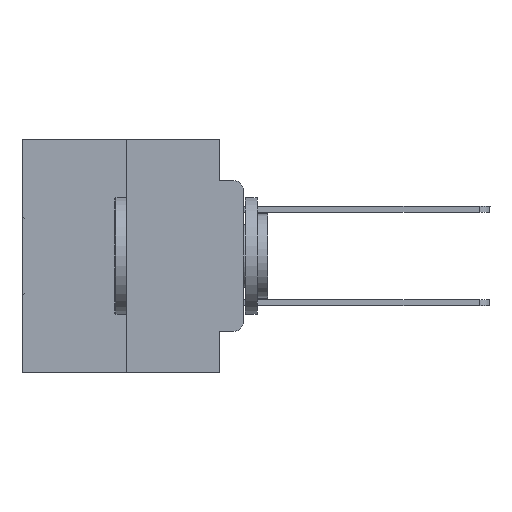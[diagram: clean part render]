
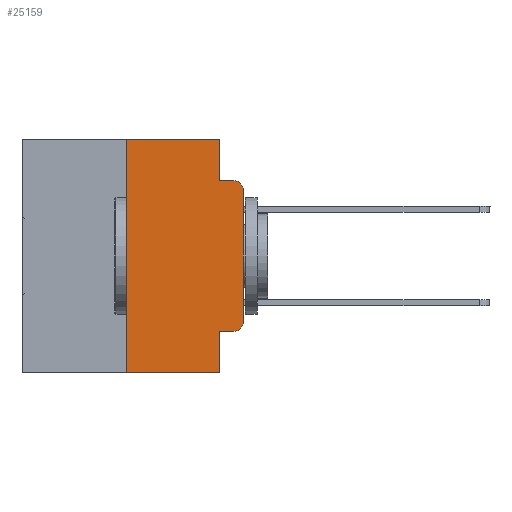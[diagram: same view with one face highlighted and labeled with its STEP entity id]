
A CAD part, left-side view. The second image highlights one B-rep face of the part: STEP entity #25159.
In plain terms, the highlighted planar face has unit normal (-1, 0, 0).
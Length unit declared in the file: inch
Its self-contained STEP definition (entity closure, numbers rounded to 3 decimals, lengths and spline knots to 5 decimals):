
#123 = ORIENTED_EDGE ( 'NONE', *, *, #10604, .T. ) ;
#193 = ORIENTED_EDGE ( 'NONE', *, *, #23013, .F. ) ;
#259 = ORIENTED_EDGE ( 'NONE', *, *, #24618, .F. ) ;
#698 = CARTESIAN_POINT ( 'NONE',  ( 0., 0., -0.3915 ) ) ;
#1073 = ORIENTED_EDGE ( 'NONE', *, *, #23435, .F. ) ;
#1440 = ORIENTED_EDGE ( 'NONE', *, *, #4378, .F. ) ;
#1446 = VERTEX_POINT ( 'NONE', #698 ) ;
#1528 = ORIENTED_EDGE ( 'NONE', *, *, #29023, .T. ) ;
#1640 = AXIS2_PLACEMENT_3D ( 'NONE', #9960, #26899, #12381 ) ;
#1668 = CARTESIAN_POINT ( 'NONE',  ( 0., 0.051, -0.4115 ) ) ;
#1795 = ORIENTED_EDGE ( 'NONE', *, *, #25644, .F. ) ;
#2915 = VERTEX_POINT ( 'NONE', #30179 ) ;
#3330 = CARTESIAN_POINT ( 'NONE',  ( 0., 0.473, 0. ) ) ;
#3555 = ORIENTED_EDGE ( 'NONE', *, *, #5461, .T. ) ;
#3593 = VERTEX_POINT ( 'NONE', #16585 ) ;
#3772 = ORIENTED_EDGE ( 'NONE', *, *, #14699, .T. ) ;
#4323 = DIRECTION ( 'NONE',  ( 0., -1., 0. ) ) ;
#4378 = EDGE_CURVE ( 'NONE', #27528, #13799, #26912, .T. ) ;
#4820 = CARTESIAN_POINT ( 'NONE',  ( 0., 0.051, -0.4115 ) ) ;
#5461 = EDGE_CURVE ( 'NONE', #28238, #3593, #11189, .T. ) ;
#5776 = DIRECTION ( 'NONE',  ( 0., -1., 0. ) ) ;
#5887 = DIRECTION ( 'NONE',  ( 0., 0., -1. ) ) ;
#6039 = DIRECTION ( 'NONE',  ( 0., 0., -1. ) ) ;
#6043 = VECTOR ( 'NONE', #5776, 39.37008 ) ;
#6338 = VECTOR ( 'NONE', #8781, 39.37008 ) ;
#6846 = DIRECTION ( 'NONE',  ( 0., -1., 0. ) ) ;
#6979 = CIRCLE ( 'NONE', #1640, 0.02 ) ;
#8599 = CARTESIAN_POINT ( 'NONE',  ( 0., 0.25, 0. ) ) ;
#8781 = DIRECTION ( 'NONE',  ( 0., 0., -1. ) ) ;
#8813 = DIRECTION ( 'NONE',  ( 0., 0., 1. ) ) ;
#9784 = FACE_OUTER_BOUND ( 'NONE', #12762, .T. ) ;
#9960 = CARTESIAN_POINT ( 'NONE',  ( 0., 0.02, -0.3915 ) ) ;
#10604 = EDGE_CURVE ( 'NONE', #21894, #22448, #30236, .T. ) ;
#10628 = CARTESIAN_POINT ( 'NONE',  ( 0., 0.473, -0.5 ) ) ;
#10688 = CARTESIAN_POINT ( 'NONE',  ( 0., 0., -0.1085 ) ) ;
#10834 = DIRECTION ( 'NONE',  ( 0., 0., 1. ) ) ;
#11189 = LINE ( 'NONE', #1668, #16890 ) ;
#11787 = LINE ( 'NONE', #22932, #23922 ) ;
#12381 = DIRECTION ( 'NONE',  ( 0., 0., -1. ) ) ;
#12550 = LINE ( 'NONE', #10628, #6043 ) ;
#12762 = EDGE_LOOP ( 'NONE', ( #30031, #123, #193, #259, #1073, #1440, #1528, #1795, #3555, #3772 ) ) ;
#13799 = VERTEX_POINT ( 'NONE', #21155 ) ;
#13917 = VECTOR ( 'NONE', #6039, 39.37008 ) ;
#14074 = VECTOR ( 'NONE', #4323, 39.37008 ) ;
#14136 = CARTESIAN_POINT ( 'NONE',  ( 0., 0.473, 0. ) ) ;
#14699 = EDGE_CURVE ( 'NONE', #3593, #1446, #6979, .T. ) ;
#14932 = CARTESIAN_POINT ( 'NONE',  ( 0., 0.02, -0.0885 ) ) ;
#14945 = CARTESIAN_POINT ( 'NONE',  ( 0., 0.02, -0.1085 ) ) ;
#16085 = CARTESIAN_POINT ( 'NONE',  ( 0., 0.25, -0.5 ) ) ;
#16376 = LINE ( 'NONE', #29285, #21309 ) ;
#16585 = CARTESIAN_POINT ( 'NONE',  ( 0., 0.02, -0.4115 ) ) ;
#16890 = VECTOR ( 'NONE', #6846, 39.37008 ) ;
#17386 = DIRECTION ( 'NONE',  ( 0., 0., -1. ) ) ;
#18207 = CARTESIAN_POINT ( 'NONE',  ( 0., 0.051, 0. ) ) ;
#18580 = AXIS2_PLACEMENT_3D ( 'NONE', #14945, #31829, #17386 ) ;
#20291 = CARTESIAN_POINT ( 'NONE',  ( 0., 0.051, -0.5 ) ) ;
#20492 = DIRECTION ( 'NONE',  ( 1., 0., 0. ) ) ;
#20515 = LINE ( 'NONE', #14136, #14074 ) ;
#20737 = CARTESIAN_POINT ( 'NONE',  ( 0., 0.051, 0. ) ) ;
#20803 = VERTEX_POINT ( 'NONE', #30848 ) ;
#21155 = CARTESIAN_POINT ( 'NONE',  ( 0., 0.25, 0. ) ) ;
#21309 = VECTOR ( 'NONE', #31678, 39.37008 ) ;
#21894 = VERTEX_POINT ( 'NONE', #10688 ) ;
#22448 = VERTEX_POINT ( 'NONE', #14932 ) ;
#22839 = PLANE ( 'NONE',  #28988 ) ;
#22932 = CARTESIAN_POINT ( 'NONE',  ( 0., 0., 0. ) ) ;
#23013 = EDGE_CURVE ( 'NONE', #2915, #22448, #16376, .T. ) ;
#23435 = EDGE_CURVE ( 'NONE', #13799, #20803, #20515, .T. ) ;
#23922 = VECTOR ( 'NONE', #10834, 39.37008 ) ;
#24618 = EDGE_CURVE ( 'NONE', #20803, #2915, #25729, .T. ) ;
#25159 = ADVANCED_FACE ( 'NONE', ( #9784 ), #22839, .F. ) ;
#25644 = EDGE_CURVE ( 'NONE', #28238, #28000, #27560, .T. ) ;
#25729 = LINE ( 'NONE', #20737, #6338 ) ;
#26153 = VECTOR ( 'NONE', #8813, 39.37008 ) ;
#26899 = DIRECTION ( 'NONE',  ( -1., 0., 0. ) ) ;
#26912 = LINE ( 'NONE', #8599, #26153 ) ;
#27528 = VERTEX_POINT ( 'NONE', #16085 ) ;
#27560 = LINE ( 'NONE', #18207, #13917 ) ;
#28000 = VERTEX_POINT ( 'NONE', #20291 ) ;
#28238 = VERTEX_POINT ( 'NONE', #4820 ) ;
#28988 = AXIS2_PLACEMENT_3D ( 'NONE', #3330, #20492, #5887 ) ;
#29023 = EDGE_CURVE ( 'NONE', #27528, #28000, #12550, .T. ) ;
#29069 = EDGE_CURVE ( 'NONE', #1446, #21894, #11787, .T. ) ;
#29285 = CARTESIAN_POINT ( 'NONE',  ( 0., 0.051, -0.0885 ) ) ;
#30031 = ORIENTED_EDGE ( 'NONE', *, *, #29069, .T. ) ;
#30179 = CARTESIAN_POINT ( 'NONE',  ( 0., 0.051, -0.0885 ) ) ;
#30236 = CIRCLE ( 'NONE', #18580, 0.02 ) ;
#30848 = CARTESIAN_POINT ( 'NONE',  ( 0., 0.051, 0. ) ) ;
#31678 = DIRECTION ( 'NONE',  ( 0., -1., 0. ) ) ;
#31829 = DIRECTION ( 'NONE',  ( -1., 0., 0. ) ) ;
